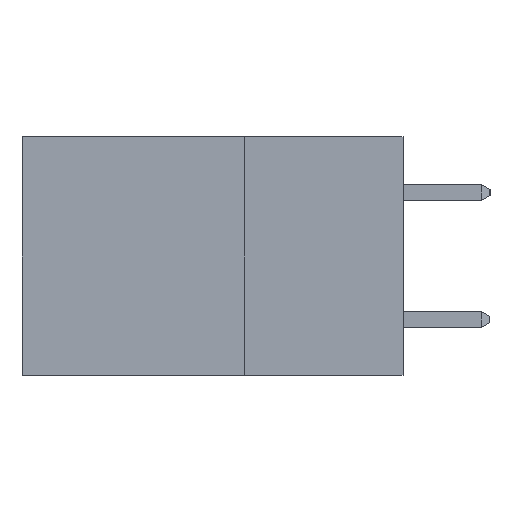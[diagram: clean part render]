
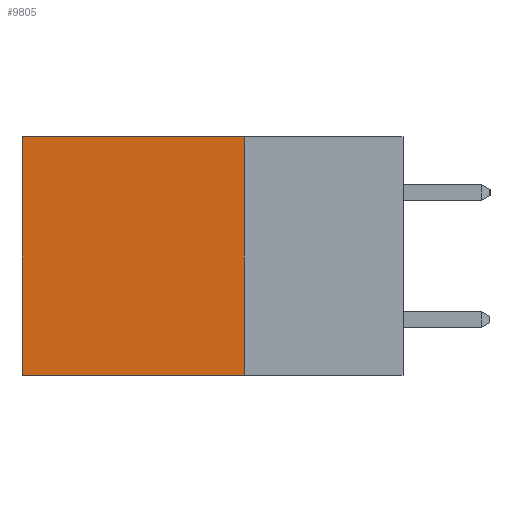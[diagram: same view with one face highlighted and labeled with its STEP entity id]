
A CAD part, left-side view. The second image highlights one B-rep face of the part: STEP entity #9805.
In plain terms, the highlighted planar face has unit normal (-1, 0, 0).
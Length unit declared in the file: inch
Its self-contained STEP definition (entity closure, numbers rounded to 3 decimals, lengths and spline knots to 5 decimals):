
#704 = CARTESIAN_POINT ( 'NONE',  ( 0.2875, 0.6, 0. ) ) ;
#757 = DIRECTION ( 'NONE',  ( 0., 0., -1. ) ) ;
#1290 = VECTOR ( 'NONE', #7710, 39.37008 ) ;
#1980 = CARTESIAN_POINT ( 'NONE',  ( 0.2875, 0.25, -0.375 ) ) ;
#2397 = DIRECTION ( 'NONE',  ( 1., 0., 0. ) ) ;
#3366 = FACE_OUTER_BOUND ( 'NONE', #8788, .T. ) ;
#4063 = ORIENTED_EDGE ( 'NONE', *, *, #13148, .F. ) ;
#4358 = LINE ( 'NONE', #12379, #5246 ) ;
#4458 = CARTESIAN_POINT ( 'NONE',  ( 0.2875, 0.6, -0.375 ) ) ;
#4786 = VECTOR ( 'NONE', #7508, 39.37008 ) ;
#4983 = VERTEX_POINT ( 'NONE', #9642 ) ;
#5190 = EDGE_CURVE ( 'NONE', #13366, #7121, #13547, .T. ) ;
#5246 = VECTOR ( 'NONE', #757, 39.37008 ) ;
#5685 = EDGE_CURVE ( 'NONE', #13366, #14598, #4358, .T. ) ;
#6735 = CARTESIAN_POINT ( 'NONE',  ( 0.2875, 0.25, -0.375 ) ) ;
#6759 = DIRECTION ( 'NONE',  ( 0., 0., -1. ) ) ;
#7121 = VERTEX_POINT ( 'NONE', #704 ) ;
#7161 = AXIS2_PLACEMENT_3D ( 'NONE', #12741, #2397, #6759 ) ;
#7508 = DIRECTION ( 'NONE',  ( 0., 1., 0. ) ) ;
#7710 = DIRECTION ( 'NONE',  ( 0., 1., 0. ) ) ;
#7894 = PLANE ( 'NONE',  #7161 ) ;
#8788 = EDGE_LOOP ( 'NONE', ( #10799, #4063, #11348, #14753 ) ) ;
#9134 = CARTESIAN_POINT ( 'NONE',  ( 0.2875, 0.25, 0. ) ) ;
#9642 = CARTESIAN_POINT ( 'NONE',  ( 0.2875, 0.6, -0.375 ) ) ;
#9722 = VECTOR ( 'NONE', #13817, 39.37008 ) ;
#9805 = ADVANCED_FACE ( 'NONE', ( #3366 ), #7894, .F. ) ;
#10657 = EDGE_CURVE ( 'NONE', #7121, #4983, #14802, .T. ) ;
#10799 = ORIENTED_EDGE ( 'NONE', *, *, #10657, .T. ) ;
#11000 = CARTESIAN_POINT ( 'NONE',  ( 0.2875, 0.25, 0. ) ) ;
#11046 = LINE ( 'NONE', #1980, #1290 ) ;
#11348 = ORIENTED_EDGE ( 'NONE', *, *, #5685, .F. ) ;
#12379 = CARTESIAN_POINT ( 'NONE',  ( 0.2875, 0.25, -0.375 ) ) ;
#12741 = CARTESIAN_POINT ( 'NONE',  ( 0.2875, 0.25, -0.375 ) ) ;
#13148 = EDGE_CURVE ( 'NONE', #14598, #4983, #11046, .T. ) ;
#13366 = VERTEX_POINT ( 'NONE', #9134 ) ;
#13547 = LINE ( 'NONE', #11000, #4786 ) ;
#13817 = DIRECTION ( 'NONE',  ( 0., 0., -1. ) ) ;
#14598 = VERTEX_POINT ( 'NONE', #6735 ) ;
#14753 = ORIENTED_EDGE ( 'NONE', *, *, #5190, .T. ) ;
#14802 = LINE ( 'NONE', #4458, #9722 ) ;
